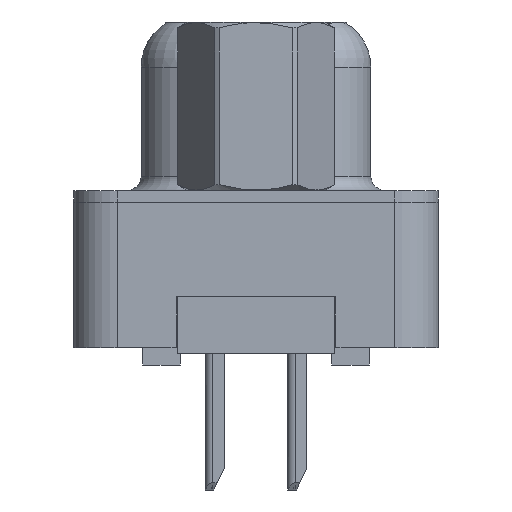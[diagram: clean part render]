
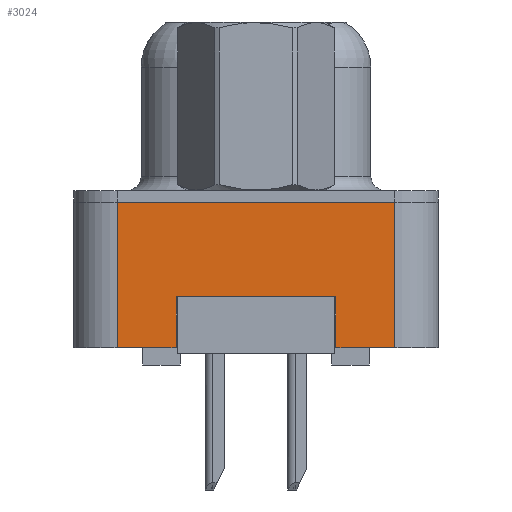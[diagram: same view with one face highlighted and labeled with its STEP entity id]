
A CAD part, left-side view. The second image highlights one B-rep face of the part: STEP entity #3024.
In plain terms, the highlighted planar face has unit normal (-1, 0, 0).
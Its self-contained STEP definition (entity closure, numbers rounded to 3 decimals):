
#252 = ORIENTED_EDGE ( 'NONE', *, *, #12185, .T. ) ;
#258 = DIRECTION ( 'NONE',  ( 0., 0., 1. ) ) ;
#286 = VERTEX_POINT ( 'NONE', #7209 ) ;
#704 = DIRECTION ( 'NONE',  ( 0., 0., -1. ) ) ;
#797 = CARTESIAN_POINT ( 'NONE',  ( -2.945, -2.75, -3.25 ) ) ;
#1041 = DIRECTION ( 'NONE',  ( 0., 1., 0. ) ) ;
#1274 = ORIENTED_EDGE ( 'NONE', *, *, #13604, .T. ) ;
#2420 = CARTESIAN_POINT ( 'NONE',  ( -2.945, -2.75, -5. ) ) ;
#2696 = CARTESIAN_POINT ( 'NONE',  ( -2.945, -4.775, -5. ) ) ;
#3024 = ADVANCED_FACE ( 'NONE', ( #14074 ), #5567, .T. ) ;
#3578 = ORIENTED_EDGE ( 'NONE', *, *, #8621, .F. ) ;
#4067 = VECTOR ( 'NONE', #19339, 1000. ) ;
#4410 = VERTEX_POINT ( 'NONE', #16930 ) ;
#4625 = EDGE_CURVE ( 'NONE', #11968, #11538, #20143, .T. ) ;
#5567 = PLANE ( 'NONE',  #12211 ) ;
#5788 = VECTOR ( 'NONE', #8572, 1000. ) ;
#5901 = LINE ( 'NONE', #17653, #4067 ) ;
#6289 = VECTOR ( 'NONE', #14660, 1000. ) ;
#6453 = VERTEX_POINT ( 'NONE', #18651 ) ;
#6492 = EDGE_CURVE ( 'NONE', #18168, #286, #16372, .T. ) ;
#6700 = VERTEX_POINT ( 'NONE', #20161 ) ;
#6772 = LINE ( 'NONE', #20086, #5788 ) ;
#7209 = CARTESIAN_POINT ( 'NONE',  ( -2.945, 2.75, -3.25 ) ) ;
#7311 = LINE ( 'NONE', #14147, #8433 ) ;
#7555 = ORIENTED_EDGE ( 'NONE', *, *, #4625, .T. ) ;
#7603 = CARTESIAN_POINT ( 'NONE',  ( -2.945, -4.775, 0. ) ) ;
#8433 = VECTOR ( 'NONE', #704, 1000. ) ;
#8572 = DIRECTION ( 'NONE',  ( 0., 0., -1. ) ) ;
#8621 = EDGE_CURVE ( 'NONE', #6700, #4410, #15901, .T. ) ;
#8722 = VECTOR ( 'NONE', #12544, 1000. ) ;
#9516 = LINE ( 'NONE', #10687, #6289 ) ;
#10687 = CARTESIAN_POINT ( 'NONE',  ( -2.945, -4.775, -5. ) ) ;
#10932 = EDGE_LOOP ( 'NONE', ( #1274, #7555, #15086, #3578, #12479, #252, #20416, #15664 ) ) ;
#11062 = EDGE_CURVE ( 'NONE', #6453, #6700, #13471, .T. ) ;
#11538 = VERTEX_POINT ( 'NONE', #18099 ) ;
#11952 = CARTESIAN_POINT ( 'NONE',  ( -2.945, -4.775, -5. ) ) ;
#11968 = VERTEX_POINT ( 'NONE', #2420 ) ;
#12185 = EDGE_CURVE ( 'NONE', #6453, #15864, #9516, .T. ) ;
#12211 = AXIS2_PLACEMENT_3D ( 'NONE', #11952, #12400, #17632 ) ;
#12400 = DIRECTION ( 'NONE',  ( -1., 0., 0. ) ) ;
#12479 = ORIENTED_EDGE ( 'NONE', *, *, #11062, .F. ) ;
#12544 = DIRECTION ( 'NONE',  ( 0., -1., 0. ) ) ;
#13471 = LINE ( 'NONE', #15586, #18035 ) ;
#13604 = EDGE_CURVE ( 'NONE', #18168, #11968, #7311, .T. ) ;
#13822 = VECTOR ( 'NONE', #21798, 1000. ) ;
#14074 = FACE_OUTER_BOUND ( 'NONE', #10932, .T. ) ;
#14147 = CARTESIAN_POINT ( 'NONE',  ( -2.945, -2.75, -3.25 ) ) ;
#14660 = DIRECTION ( 'NONE',  ( 0., -1., 0. ) ) ;
#15086 = ORIENTED_EDGE ( 'NONE', *, *, #20306, .T. ) ;
#15586 = CARTESIAN_POINT ( 'NONE',  ( -2.945, 4.775, -5. ) ) ;
#15664 = ORIENTED_EDGE ( 'NONE', *, *, #6492, .F. ) ;
#15864 = VERTEX_POINT ( 'NONE', #16732 ) ;
#15901 = LINE ( 'NONE', #7603, #8722 ) ;
#16372 = LINE ( 'NONE', #18263, #20285 ) ;
#16732 = CARTESIAN_POINT ( 'NONE',  ( -2.945, 2.75, -5. ) ) ;
#16930 = CARTESIAN_POINT ( 'NONE',  ( -2.945, -4.775, 0. ) ) ;
#17632 = DIRECTION ( 'NONE',  ( 0., 0., 1. ) ) ;
#17653 = CARTESIAN_POINT ( 'NONE',  ( -2.945, -4.775, -5. ) ) ;
#18035 = VECTOR ( 'NONE', #258, 1000. ) ;
#18099 = CARTESIAN_POINT ( 'NONE',  ( -2.945, -4.775, -5. ) ) ;
#18168 = VERTEX_POINT ( 'NONE', #797 ) ;
#18263 = CARTESIAN_POINT ( 'NONE',  ( -2.945, 2.75, -3.25 ) ) ;
#18651 = CARTESIAN_POINT ( 'NONE',  ( -2.945, 4.775, -5. ) ) ;
#18772 = EDGE_CURVE ( 'NONE', #286, #15864, #6772, .T. ) ;
#19339 = DIRECTION ( 'NONE',  ( 0., 0., 1. ) ) ;
#20086 = CARTESIAN_POINT ( 'NONE',  ( -2.945, 2.75, -3.25 ) ) ;
#20143 = LINE ( 'NONE', #2696, #13822 ) ;
#20161 = CARTESIAN_POINT ( 'NONE',  ( -2.945, 4.775, 0. ) ) ;
#20285 = VECTOR ( 'NONE', #1041, 1000. ) ;
#20306 = EDGE_CURVE ( 'NONE', #11538, #4410, #5901, .T. ) ;
#20416 = ORIENTED_EDGE ( 'NONE', *, *, #18772, .F. ) ;
#21798 = DIRECTION ( 'NONE',  ( 0., -1., 0. ) ) ;
